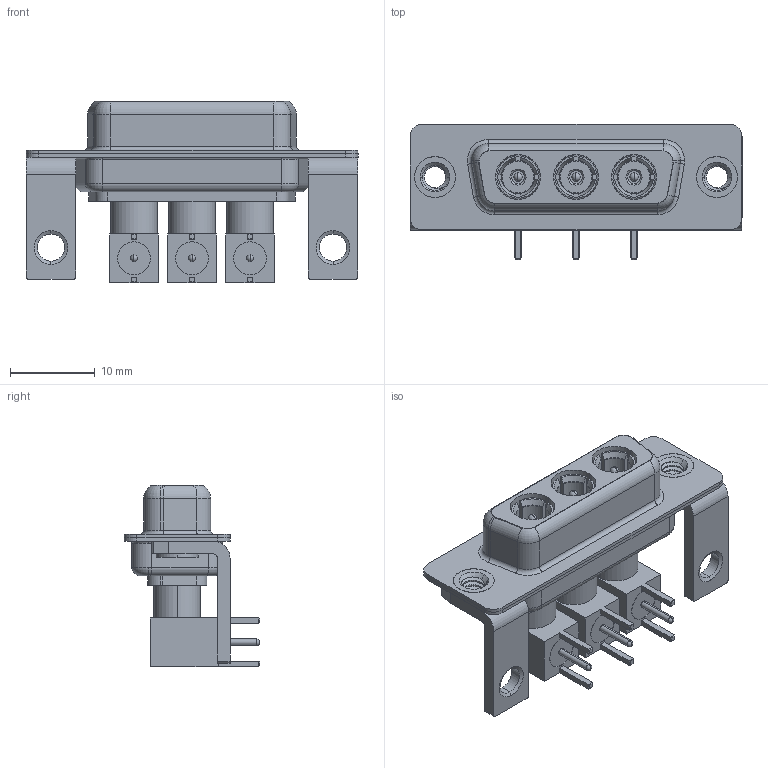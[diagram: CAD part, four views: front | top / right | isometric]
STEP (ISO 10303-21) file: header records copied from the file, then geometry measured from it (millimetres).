
FILE_DESCRIPTION (( 'STEP AP203' ), '1' );
FILE_NAME ('630-3W3-240-7NC.STEP', '2022-05-27T16:45:51', ( '' ), ( '' ), 'SwSTEP 2.0', 'SolidWorks 2020', '' );
FILE_SCHEMA (( 'CONFIG_CONTROL_DESIGN' ));
Length unit declared in the file: millimetre
Products named in the file (15): Co-Ax Plug_RA PC Tail; Co-Ax Plug Assy_RA; Insulator Pin_Straight PC Tail; 630Combo Housing_3W3; 630-3W3-240-7NC; Insulator RA Pin; 630Combo Threaded Rivet_B; RA Back Shell; 630Combo Shell Front_15 Contacts; Locking Collar; 630Combo Stabilizer Bracket; 630Combo Shell Rear_15 Contacts; Pin_RA
Assembly tree (28 placements, depth 3):
  630-3W3-240-7NC
    630Combo Housing_3W3
    630Combo Shell Front_15 Contacts
    630Combo Shell Rear_15 Contacts
    630Combo Threaded Rivet_B  x2
    630Combo Stabilizer Bracket  x2
    Co-Ax Plug Assy_RA
      Co-Ax Plug_RA PC Tail
      Insulator Pin_Straight PC Tail
      Pin_RA
      Locking Collar
      RA Back Shell
      Insulator RA Pin
    Co-Ax Plug Assy_RA
      Co-Ax Plug_RA PC Tail
      Insulator Pin_Straight PC Tail
      Pin_RA
      Locking Collar
      RA Back Shell
      Insulator RA Pin
    Co-Ax Plug Assy_RA
      Co-Ax Plug_RA PC Tail
      Insulator Pin_Straight PC Tail
      Pin_RA
      Locking Collar
      RA Back Shell
      Insulator RA Pin
Bounding box: 39.2 x 16 x 21.41 mm (x, y, z)
Volume: 3401.5 mm3; surface area: 8377.3 mm2
Topology: 25 solids, 25 shells, 821 faces, 1988 edges, 1246 vertices
Faces by surface type: cylinder 350, plane 288, cone 87, torus 75, sphere 12, bspline 9
Entity records: 16717 total; most frequent: CARTESIAN_POINT 4060, DIRECTION 2415, ORIENTED_EDGE 2134, EDGE_CURVE 1067, AXIS2_PLACEMENT_3D 970, VERTEX_POINT 673, EDGE_LOOP 502, CIRCLE 497
